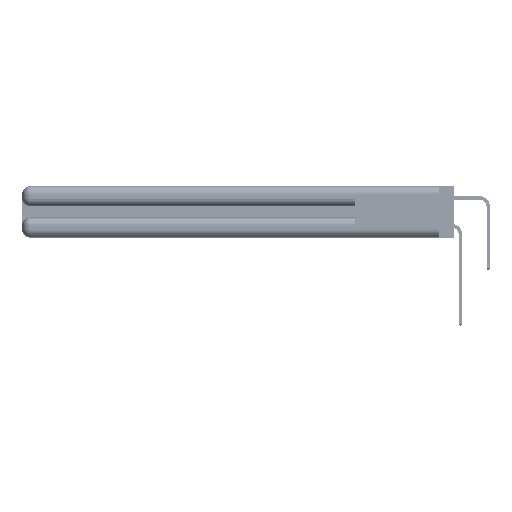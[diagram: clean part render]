
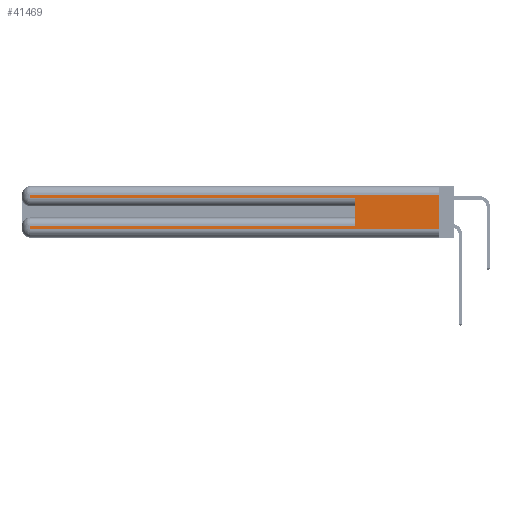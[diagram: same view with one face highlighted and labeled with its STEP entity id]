
A CAD part, left-side view. The second image highlights one B-rep face of the part: STEP entity #41469.
In plain terms, the highlighted planar face has unit normal (-1, 0, 0).
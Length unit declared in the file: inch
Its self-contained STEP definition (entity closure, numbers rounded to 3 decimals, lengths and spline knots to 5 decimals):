
#2798 = CARTESIAN_POINT ( 'NONE',  ( 0., 0., 0.06 ) ) ;
#4269 = DIRECTION ( 'NONE',  ( 0., 1., 0. ) ) ;
#6493 = CARTESIAN_POINT ( 'NONE',  ( 0., 0., 0.31 ) ) ;
#7284 = DIRECTION ( 'NONE',  ( 0., 1., 0. ) ) ;
#8203 = EDGE_CURVE ( 'NONE', #31734, #17343, #26712, .T. ) ;
#8207 = DIRECTION ( 'NONE',  ( 0., 0., -1. ) ) ;
#8454 = CARTESIAN_POINT ( 'NONE',  ( 0., 2.94, 0.37 ) ) ;
#8650 = FACE_OUTER_BOUND ( 'NONE', #18573, .T. ) ;
#9388 = CARTESIAN_POINT ( 'NONE',  ( 0., 0., 0.085 ) ) ;
#9869 = DIRECTION ( 'NONE',  ( 0., 0., -1. ) ) ;
#13620 = VECTOR ( 'NONE', #54356, 39.37008 ) ;
#14415 = ORIENTED_EDGE ( 'NONE', *, *, #8203, .F. ) ;
#16839 = PLANE ( 'NONE',  #33905 ) ;
#17343 = VERTEX_POINT ( 'NONE', #52367 ) ;
#17633 = CARTESIAN_POINT ( 'NONE',  ( 0., 2.94, 0.37 ) ) ;
#17869 = VECTOR ( 'NONE', #35000, 39.37008 ) ;
#18555 = ORIENTED_EDGE ( 'NONE', *, *, #20091, .T. ) ;
#18573 = EDGE_LOOP ( 'NONE', ( #53718, #18555, #18831, #25680, #14415, #41126, #52291, #43069 ) ) ;
#18831 = ORIENTED_EDGE ( 'NONE', *, *, #20289, .T. ) ;
#19270 = VERTEX_POINT ( 'NONE', #30937 ) ;
#20091 = EDGE_CURVE ( 'NONE', #22004, #19270, #49069, .T. ) ;
#20289 = EDGE_CURVE ( 'NONE', #19270, #25001, #43359, .T. ) ;
#21529 = CARTESIAN_POINT ( 'NONE',  ( 0., 0., 0.37 ) ) ;
#21630 = VERTEX_POINT ( 'NONE', #46524 ) ;
#22004 = VERTEX_POINT ( 'NONE', #50030 ) ;
#22173 = LINE ( 'NONE', #45835, #56591 ) ;
#22830 = EDGE_CURVE ( 'NONE', #22004, #25527, #22173, .T. ) ;
#23963 = CARTESIAN_POINT ( 'NONE',  ( 0., 0.6, 0.145 ) ) ;
#25001 = VERTEX_POINT ( 'NONE', #40119 ) ;
#25527 = VERTEX_POINT ( 'NONE', #39855 ) ;
#25680 = ORIENTED_EDGE ( 'NONE', *, *, #52163, .T. ) ;
#26712 = LINE ( 'NONE', #23963, #33016 ) ;
#27138 = LINE ( 'NONE', #30020, #51744 ) ;
#28357 = VERTEX_POINT ( 'NONE', #41360 ) ;
#30020 = CARTESIAN_POINT ( 'NONE',  ( 0., 0., 0.285 ) ) ;
#30937 = CARTESIAN_POINT ( 'NONE',  ( 0., 2.94, 0.31 ) ) ;
#31244 = LINE ( 'NONE', #2798, #17869 ) ;
#31734 = VERTEX_POINT ( 'NONE', #47540 ) ;
#33016 = VECTOR ( 'NONE', #37541, 39.37008 ) ;
#33905 = AXIS2_PLACEMENT_3D ( 'NONE', #21529, #52975, #8207 ) ;
#35000 = DIRECTION ( 'NONE',  ( 0., -1., 0. ) ) ;
#37541 = DIRECTION ( 'NONE',  ( 0., 0., 1. ) ) ;
#39088 = DIRECTION ( 'NONE',  ( 0., -1., 0. ) ) ;
#39855 = CARTESIAN_POINT ( 'NONE',  ( 0., 0., 0.06 ) ) ;
#40119 = CARTESIAN_POINT ( 'NONE',  ( 0., 2.94, 0.285 ) ) ;
#40366 = LINE ( 'NONE', #9388, #41745 ) ;
#41126 = ORIENTED_EDGE ( 'NONE', *, *, #54236, .T. ) ;
#41360 = CARTESIAN_POINT ( 'NONE',  ( 0., 2.94, 0.06 ) ) ;
#41469 = ADVANCED_FACE ( 'NONE', ( #8650 ), #16839, .F. ) ;
#41745 = VECTOR ( 'NONE', #4269, 39.37008 ) ;
#43069 = ORIENTED_EDGE ( 'NONE', *, *, #53263, .T. ) ;
#43359 = LINE ( 'NONE', #8454, #50427 ) ;
#43833 = LINE ( 'NONE', #17633, #13620 ) ;
#45835 = CARTESIAN_POINT ( 'NONE',  ( 0., 0., 0.37 ) ) ;
#46524 = CARTESIAN_POINT ( 'NONE',  ( 0., 2.94, 0.085 ) ) ;
#47540 = CARTESIAN_POINT ( 'NONE',  ( 0., 0.6, 0.085 ) ) ;
#48326 = DIRECTION ( 'NONE',  ( 0., 0., -1. ) ) ;
#49069 = LINE ( 'NONE', #6493, #52553 ) ;
#50030 = CARTESIAN_POINT ( 'NONE',  ( 0., 0., 0.31 ) ) ;
#50427 = VECTOR ( 'NONE', #48326, 39.37008 ) ;
#50547 = EDGE_CURVE ( 'NONE', #21630, #28357, #43833, .T. ) ;
#51744 = VECTOR ( 'NONE', #39088, 39.37008 ) ;
#52163 = EDGE_CURVE ( 'NONE', #25001, #17343, #27138, .T. ) ;
#52291 = ORIENTED_EDGE ( 'NONE', *, *, #50547, .T. ) ;
#52367 = CARTESIAN_POINT ( 'NONE',  ( 0., 0.6, 0.285 ) ) ;
#52553 = VECTOR ( 'NONE', #7284, 39.37008 ) ;
#52975 = DIRECTION ( 'NONE',  ( 1., 0., 0. ) ) ;
#53263 = EDGE_CURVE ( 'NONE', #28357, #25527, #31244, .T. ) ;
#53718 = ORIENTED_EDGE ( 'NONE', *, *, #22830, .F. ) ;
#54236 = EDGE_CURVE ( 'NONE', #31734, #21630, #40366, .T. ) ;
#54356 = DIRECTION ( 'NONE',  ( 0., 0., -1. ) ) ;
#56591 = VECTOR ( 'NONE', #9869, 39.37008 ) ;
